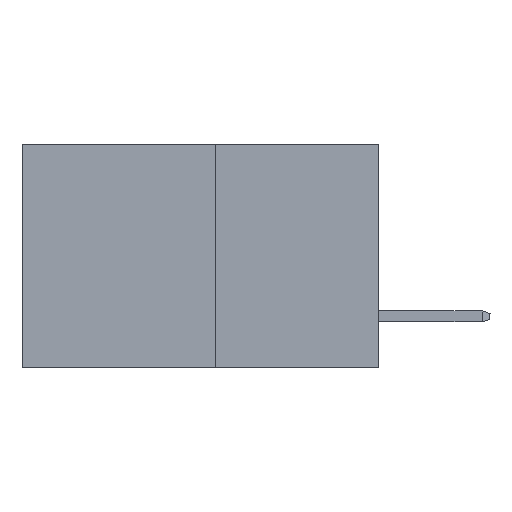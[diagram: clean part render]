
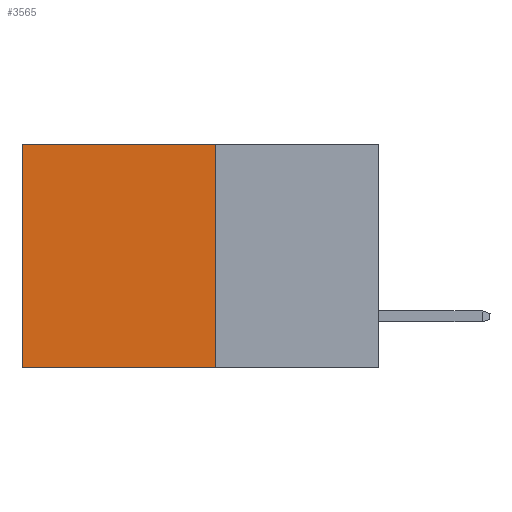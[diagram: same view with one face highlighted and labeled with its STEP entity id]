
A CAD part, left-side view. The second image highlights one B-rep face of the part: STEP entity #3565.
In plain terms, the highlighted planar face has unit normal (-1, 0, 0).
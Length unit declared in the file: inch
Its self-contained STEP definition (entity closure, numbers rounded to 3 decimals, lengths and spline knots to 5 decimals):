
#824 = CARTESIAN_POINT ( 'NONE',  ( 0.277, 0.27, -0.37 ) ) ;
#1223 = CARTESIAN_POINT ( 'NONE',  ( 0.277, 0.27, 0. ) ) ;
#1573 = VERTEX_POINT ( 'NONE', #16100 ) ;
#1743 = VECTOR ( 'NONE', #10878, 39.37008 ) ;
#3297 = VERTEX_POINT ( 'NONE', #3815 ) ;
#3565 = ADVANCED_FACE ( 'NONE', ( #4502 ), #13268, .F. ) ;
#3709 = DIRECTION ( 'NONE',  ( 0., 0., -1. ) ) ;
#3815 = CARTESIAN_POINT ( 'NONE',  ( 0.277, 0.59, 0. ) ) ;
#4143 = EDGE_CURVE ( 'NONE', #8062, #1573, #15263, .T. ) ;
#4502 = FACE_OUTER_BOUND ( 'NONE', #6308, .T. ) ;
#4870 = ORIENTED_EDGE ( 'NONE', *, *, #15205, .F. ) ;
#5727 = DIRECTION ( 'NONE',  ( 0., 1., 0. ) ) ;
#5888 = ORIENTED_EDGE ( 'NONE', *, *, #11573, .T. ) ;
#6292 = EDGE_CURVE ( 'NONE', #3297, #1573, #12866, .T. ) ;
#6308 = EDGE_LOOP ( 'NONE', ( #13919, #13634, #4870, #5888 ) ) ;
#7517 = LINE ( 'NONE', #824, #10085 ) ;
#8062 = VERTEX_POINT ( 'NONE', #14610 ) ;
#8389 = CARTESIAN_POINT ( 'NONE',  ( 0.277, 0.27, 0. ) ) ;
#8601 = VECTOR ( 'NONE', #5727, 39.37008 ) ;
#8640 = LINE ( 'NONE', #8389, #1743 ) ;
#10085 = VECTOR ( 'NONE', #12367, 39.37008 ) ;
#10878 = DIRECTION ( 'NONE',  ( 0., 1., 0. ) ) ;
#11573 = EDGE_CURVE ( 'NONE', #15392, #3297, #8640, .T. ) ;
#11654 = AXIS2_PLACEMENT_3D ( 'NONE', #13482, #13628, #13639 ) ;
#11774 = CARTESIAN_POINT ( 'NONE',  ( 0.277, 0.27, -0.37 ) ) ;
#12367 = DIRECTION ( 'NONE',  ( 0., 0., -1. ) ) ;
#12866 = LINE ( 'NONE', #13795, #16166 ) ;
#13268 = PLANE ( 'NONE',  #11654 ) ;
#13482 = CARTESIAN_POINT ( 'NONE',  ( 0.277, 0.27, -0.37 ) ) ;
#13628 = DIRECTION ( 'NONE',  ( 1., 0., 0. ) ) ;
#13634 = ORIENTED_EDGE ( 'NONE', *, *, #4143, .F. ) ;
#13639 = DIRECTION ( 'NONE',  ( 0., 0., -1. ) ) ;
#13795 = CARTESIAN_POINT ( 'NONE',  ( 0.277, 0.59, -0.37 ) ) ;
#13919 = ORIENTED_EDGE ( 'NONE', *, *, #6292, .T. ) ;
#14610 = CARTESIAN_POINT ( 'NONE',  ( 0.277, 0.27, -0.37 ) ) ;
#15205 = EDGE_CURVE ( 'NONE', #15392, #8062, #7517, .T. ) ;
#15263 = LINE ( 'NONE', #11774, #8601 ) ;
#15392 = VERTEX_POINT ( 'NONE', #1223 ) ;
#16100 = CARTESIAN_POINT ( 'NONE',  ( 0.277, 0.59, -0.37 ) ) ;
#16166 = VECTOR ( 'NONE', #3709, 39.37008 ) ;
